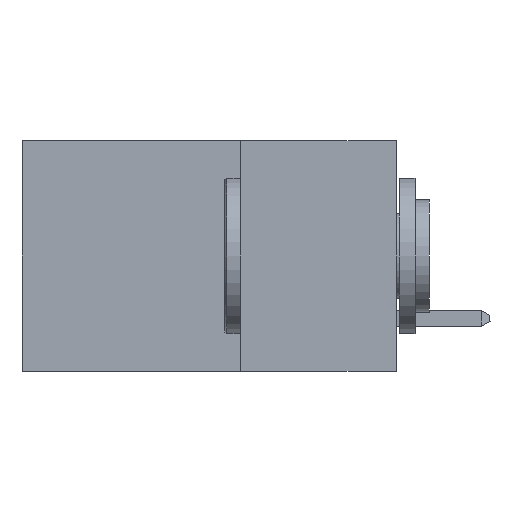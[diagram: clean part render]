
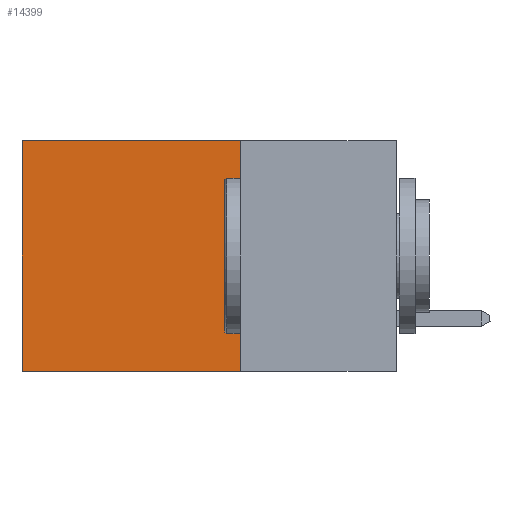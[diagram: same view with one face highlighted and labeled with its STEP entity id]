
A CAD part, left-side view. The second image highlights one B-rep face of the part: STEP entity #14399.
In plain terms, the highlighted planar face has unit normal (-1, 0, 0).
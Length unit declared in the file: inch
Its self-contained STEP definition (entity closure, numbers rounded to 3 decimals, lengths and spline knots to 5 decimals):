
#85 = VERTEX_POINT ( 'NONE', #5675 ) ;
#356 = ORIENTED_EDGE ( 'NONE', *, *, #5642, .T. ) ;
#1192 = VECTOR ( 'NONE', #6731, 39.37008 ) ;
#2354 = VERTEX_POINT ( 'NONE', #15071 ) ;
#3562 = CARTESIAN_POINT ( 'NONE',  ( 0.298, 0.6, 0. ) ) ;
#3802 = DIRECTION ( 'NONE',  ( 1., 0., 0. ) ) ;
#5642 = EDGE_CURVE ( 'NONE', #85, #2354, #11311, .T. ) ;
#5675 = CARTESIAN_POINT ( 'NONE',  ( 0.298, 0.6, 0. ) ) ;
#6181 = DIRECTION ( 'NONE',  ( 0., 1., 0. ) ) ;
#6195 = ORIENTED_EDGE ( 'NONE', *, *, #18632, .T. ) ;
#6731 = DIRECTION ( 'NONE',  ( 0., 0., -1. ) ) ;
#8465 = DIRECTION ( 'NONE',  ( 0., 0., -1. ) ) ;
#8643 = PLANE ( 'NONE',  #17597 ) ;
#10027 = LINE ( 'NONE', #19439, #16230 ) ;
#11288 = VERTEX_POINT ( 'NONE', #14109 ) ;
#11311 = LINE ( 'NONE', #3562, #1192 ) ;
#11526 = CARTESIAN_POINT ( 'NONE',  ( 0.298, 0.25, 0. ) ) ;
#12857 = ORIENTED_EDGE ( 'NONE', *, *, #13185, .F. ) ;
#13185 = EDGE_CURVE ( 'NONE', #17393, #11288, #20415, .T. ) ;
#14109 = CARTESIAN_POINT ( 'NONE',  ( 0.298, 0.25, -0.37 ) ) ;
#14128 = EDGE_CURVE ( 'NONE', #11288, #2354, #10027, .T. ) ;
#14399 = ADVANCED_FACE ( 'NONE', ( #20109 ), #8643, .F. ) ;
#15071 = CARTESIAN_POINT ( 'NONE',  ( 0.298, 0.6, -0.37 ) ) ;
#15841 = LINE ( 'NONE', #17972, #19174 ) ;
#16230 = VECTOR ( 'NONE', #6181, 39.37008 ) ;
#16983 = CARTESIAN_POINT ( 'NONE',  ( 0.298, 0.25, 0. ) ) ;
#17393 = VERTEX_POINT ( 'NONE', #11526 ) ;
#17511 = ORIENTED_EDGE ( 'NONE', *, *, #14128, .F. ) ;
#17597 = AXIS2_PLACEMENT_3D ( 'NONE', #16983, #3802, #20094 ) ;
#17657 = EDGE_LOOP ( 'NONE', ( #356, #17511, #12857, #6195 ) ) ;
#17901 = DIRECTION ( 'NONE',  ( 0., 1., 0. ) ) ;
#17972 = CARTESIAN_POINT ( 'NONE',  ( 0.298, 0.25, 0. ) ) ;
#18399 = CARTESIAN_POINT ( 'NONE',  ( 0.298, 0.25, 0. ) ) ;
#18632 = EDGE_CURVE ( 'NONE', #17393, #85, #15841, .T. ) ;
#19174 = VECTOR ( 'NONE', #17901, 39.37008 ) ;
#19361 = VECTOR ( 'NONE', #8465, 39.37008 ) ;
#19439 = CARTESIAN_POINT ( 'NONE',  ( 0.298, 0.25, -0.37 ) ) ;
#20094 = DIRECTION ( 'NONE',  ( 0., 0., -1. ) ) ;
#20109 = FACE_OUTER_BOUND ( 'NONE', #17657, .T. ) ;
#20415 = LINE ( 'NONE', #18399, #19361 ) ;
